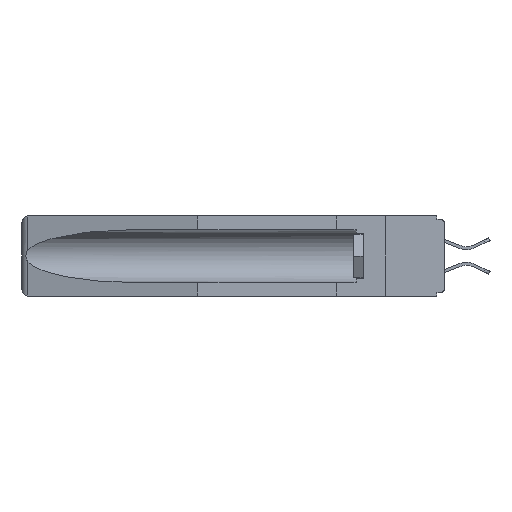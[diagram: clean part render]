
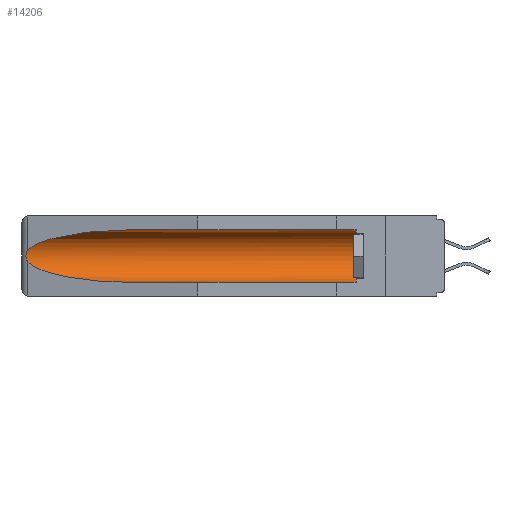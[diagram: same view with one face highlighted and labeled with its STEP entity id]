
A CAD part, left-side view. The second image highlights one B-rep face of the part: STEP entity #14206.
In plain terms, the highlighted cylindrical face has radius 2.857 mm (diameter 5.715 mm), a partial arc.
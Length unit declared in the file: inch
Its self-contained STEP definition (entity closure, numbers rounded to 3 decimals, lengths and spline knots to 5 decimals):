
#422 = VERTEX_POINT ( 'NONE', #19449 ) ;
#877 = EDGE_CURVE ( 'NONE', #6329, #7833, #1854, .T. ) ;
#1045 = CARTESIAN_POINT ( 'NONE',  ( 0.155, -0.30754, -0.059 ) ) ;
#1189 = EDGE_CURVE ( 'NONE', #7833, #20120, #15866, .T. ) ;
#1605 = VERTEX_POINT ( 'NONE', #11071 ) ;
#1854 = CIRCLE ( 'NONE', #20347, 0.1125 ) ;
#2019 = ORIENTED_EDGE ( 'NONE', *, *, #13442, .T. ) ;
#2357 = CARTESIAN_POINT ( 'NONE',  ( 0.21114, 1.30732, -0.059 ) ) ;
#2978 = CARTESIAN_POINT ( 'NONE',  ( 0.2675, 1.53308, -0.16763 ) ) ;
#3626 = DIRECTION ( 'NONE',  ( 0., 0., 1. ) ) ;
#4050 = VERTEX_POINT ( 'NONE', #18329 ) ;
#5938 = ORIENTED_EDGE ( 'NONE', *, *, #1189, .T. ) ;
#6118 = AXIS2_PLACEMENT_3D ( 'NONE', #8466, #10234, #3626 ) ;
#6184 = CARTESIAN_POINT ( 'NONE',  ( 0.26537, 1.52718, -0.19328 ) ) ;
#6265 = LINE ( 'NONE', #15452, #12352 ) ;
#6329 = VERTEX_POINT ( 'NONE', #16186 ) ;
#6530 = B_SPLINE_CURVE_WITH_KNOTS ( 'NONE', 3,
 ( #18707, #20373, #9037, #15459, #2978, #14078, #21015, #11101, #19208, #6184 ),
 .UNSPECIFIED., .F., .F.,
 ( 4, 2, 2, 2, 4 ),
 ( 0., 0.00029, 0.00058, 0.00087, 0.00117 ),
 .UNSPECIFIED. ) ;
#6784 =( BOUNDED_CURVE ( )  B_SPLINE_CURVE ( 3, ( #15199, #2357, #12089, #20451 ),
 .UNSPECIFIED., .F., .F. ) 
 B_SPLINE_CURVE_WITH_KNOTS ( ( 4, 4 ),
 ( 4.71239, 6.08839 ),
 .UNSPECIFIED. ) 
 CURVE ( )  GEOMETRIC_REPRESENTATION_ITEM ( )  RATIONAL_B_SPLINE_CURVE ( ( 1., 0.848, 0.848, 1. ) ) 
 REPRESENTATION_ITEM ( '' )  );
#7011 = ORIENTED_EDGE ( 'NONE', *, *, #10335, .T. ) ;
#7459 = EDGE_CURVE ( 'NONE', #6329, #4050, #6265, .T. ) ;
#7833 = VERTEX_POINT ( 'NONE', #18440 ) ;
#8230 = CARTESIAN_POINT ( 'NONE',  ( 0.155, 0.126, -0.1715 ) ) ;
#8466 = CARTESIAN_POINT ( 'NONE',  ( 0.155, -0.30754, -0.1715 ) ) ;
#8534 = ORIENTED_EDGE ( 'NONE', *, *, #877, .T. ) ;
#8953 = DIRECTION ( 'NONE',  ( 0., 1., 0. ) ) ;
#9037 = CARTESIAN_POINT ( 'NONE',  ( 0.26654, 1.53092, -0.15636 ) ) ;
#9859 = DIRECTION ( 'NONE',  ( 0., 0., 1. ) ) ;
#9981 = VECTOR ( 'NONE', #19089, 39.37008 ) ;
#10234 = DIRECTION ( 'NONE',  ( 0., 1., 0. ) ) ;
#10335 = EDGE_CURVE ( 'NONE', #20120, #1605, #6784, .T. ) ;
#10832 = CYLINDRICAL_SURFACE ( 'NONE', #6118, 0.1125 ) ;
#11071 = CARTESIAN_POINT ( 'NONE',  ( 0.26537, 1.52718, -0.14972 ) ) ;
#11101 = CARTESIAN_POINT ( 'NONE',  ( 0.26655, 1.53094, -0.18657 ) ) ;
#11866 =( BOUNDED_CURVE ( )  B_SPLINE_CURVE ( 3, ( #15322, #13408, #18439, #18571 ),
 .UNSPECIFIED., .F., .F. ) 
 B_SPLINE_CURVE_WITH_KNOTS ( ( 4, 4 ),
 ( 0.1948, 1.5708 ),
 .UNSPECIFIED. ) 
 CURVE ( )  GEOMETRIC_REPRESENTATION_ITEM ( )  RATIONAL_B_SPLINE_CURVE ( ( 1., 0.848, 0.848, 1. ) ) 
 REPRESENTATION_ITEM ( '' )  );
#12089 = CARTESIAN_POINT ( 'NONE',  ( 0.25451, 1.48313, -0.09465 ) ) ;
#12181 = ORIENTED_EDGE ( 'NONE', *, *, #14800, .T. ) ;
#12352 = VECTOR ( 'NONE', #8953, 39.37008 ) ;
#13408 = CARTESIAN_POINT ( 'NONE',  ( 0.25451, 1.48313, -0.24835 ) ) ;
#13442 = EDGE_CURVE ( 'NONE', #422, #4050, #11866, .T. ) ;
#14078 = CARTESIAN_POINT ( 'NONE',  ( 0.2675, 1.53308, -0.17534 ) ) ;
#14206 = ADVANCED_FACE ( 'NONE', ( #18677 ), #10832, .F. ) ;
#14800 = EDGE_CURVE ( 'NONE', #1605, #422, #6530, .T. ) ;
#15199 = CARTESIAN_POINT ( 'NONE',  ( 0.155, 1.07973, -0.059 ) ) ;
#15322 = CARTESIAN_POINT ( 'NONE',  ( 0.26537, 1.52718, -0.19328 ) ) ;
#15452 = CARTESIAN_POINT ( 'NONE',  ( 0.155, -0.30754, -0.284 ) ) ;
#15459 = CARTESIAN_POINT ( 'NONE',  ( 0.2673, 1.5327, -0.16383 ) ) ;
#15866 = LINE ( 'NONE', #1045, #9981 ) ;
#16186 = CARTESIAN_POINT ( 'NONE',  ( 0.155, 0.126, -0.284 ) ) ;
#18067 = EDGE_LOOP ( 'NONE', ( #7011, #12181, #2019, #19917, #8534, #5938 ) ) ;
#18329 = CARTESIAN_POINT ( 'NONE',  ( 0.155, 1.07973, -0.284 ) ) ;
#18439 = CARTESIAN_POINT ( 'NONE',  ( 0.21114, 1.30732, -0.284 ) ) ;
#18440 = CARTESIAN_POINT ( 'NONE',  ( 0.155, 0.126, -0.059 ) ) ;
#18571 = CARTESIAN_POINT ( 'NONE',  ( 0.155, 1.07973, -0.284 ) ) ;
#18677 = FACE_OUTER_BOUND ( 'NONE', #18067, .T. ) ;
#18707 = CARTESIAN_POINT ( 'NONE',  ( 0.26537, 1.52718, -0.14972 ) ) ;
#19089 = DIRECTION ( 'NONE',  ( 0., 1., 0. ) ) ;
#19208 = CARTESIAN_POINT ( 'NONE',  ( 0.26597, 1.5296, -0.19026 ) ) ;
#19449 = CARTESIAN_POINT ( 'NONE',  ( 0.26537, 1.52718, -0.19328 ) ) ;
#19713 = DIRECTION ( 'NONE',  ( 0., -1., 0. ) ) ;
#19917 = ORIENTED_EDGE ( 'NONE', *, *, #7459, .F. ) ;
#20120 = VERTEX_POINT ( 'NONE', #21233 ) ;
#20347 = AXIS2_PLACEMENT_3D ( 'NONE', #8230, #19713, #9859 ) ;
#20373 = CARTESIAN_POINT ( 'NONE',  ( 0.26597, 1.52961, -0.15275 ) ) ;
#20451 = CARTESIAN_POINT ( 'NONE',  ( 0.26537, 1.52718, -0.14972 ) ) ;
#21015 = CARTESIAN_POINT ( 'NONE',  ( 0.2673, 1.53269, -0.17917 ) ) ;
#21233 = CARTESIAN_POINT ( 'NONE',  ( 0.155, 1.07973, -0.059 ) ) ;
